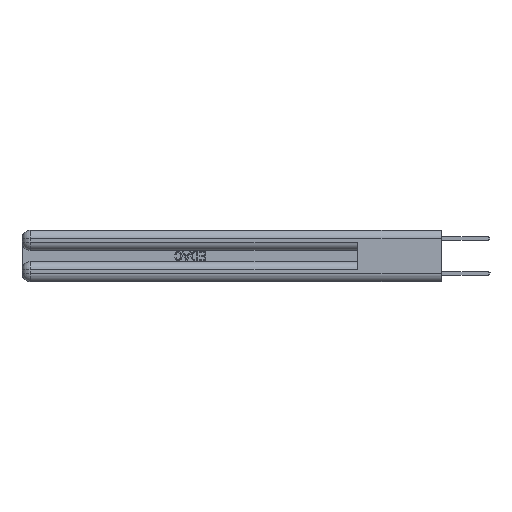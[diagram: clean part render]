
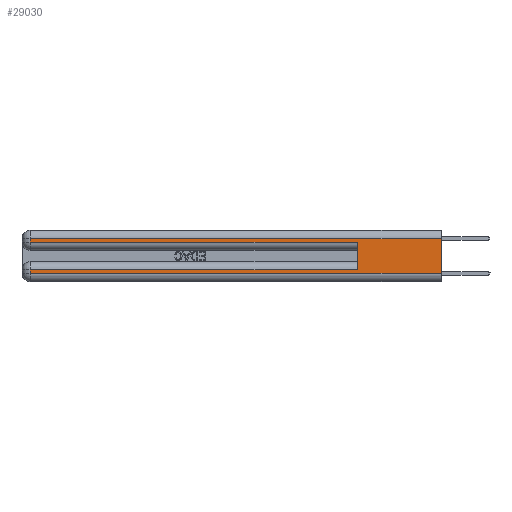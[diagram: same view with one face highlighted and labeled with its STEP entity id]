
A CAD part, left-side view. The second image highlights one B-rep face of the part: STEP entity #29030.
In plain terms, the highlighted planar face has unit normal (-1, 0, 0).
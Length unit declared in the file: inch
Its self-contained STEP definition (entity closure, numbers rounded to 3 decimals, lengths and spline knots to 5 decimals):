
#73 = EDGE_CURVE ( 'NONE', #23236, #11165, #15720, .T. ) ;
#174 = LINE ( 'NONE', #9758, #1779 ) ;
#1779 = VECTOR ( 'NONE', #19811, 39.37008 ) ;
#2543 = VERTEX_POINT ( 'NONE', #21109 ) ;
#2644 = CARTESIAN_POINT ( 'NONE',  ( 0., 2.94, 0.31 ) ) ;
#2807 = ORIENTED_EDGE ( 'NONE', *, *, #21782, .T. ) ;
#2989 = LINE ( 'NONE', #7926, #9558 ) ;
#2991 = DIRECTION ( 'NONE',  ( 0., -1., 0. ) ) ;
#3106 = VECTOR ( 'NONE', #4340, 39.37008 ) ;
#3146 = CARTESIAN_POINT ( 'NONE',  ( 0., 0., 0.37 ) ) ;
#3675 = EDGE_CURVE ( 'NONE', #23907, #11270, #6898, .T. ) ;
#4340 = DIRECTION ( 'NONE',  ( 0., 0., 1. ) ) ;
#4606 = LINE ( 'NONE', #21696, #10501 ) ;
#4812 = CARTESIAN_POINT ( 'NONE',  ( 0., 0., 0.06 ) ) ;
#5123 = AXIS2_PLACEMENT_3D ( 'NONE', #3146, #22625, #29956 ) ;
#6491 = ORIENTED_EDGE ( 'NONE', *, *, #29100, .T. ) ;
#6836 = VECTOR ( 'NONE', #2991, 39.37008 ) ;
#6898 = LINE ( 'NONE', #23993, #3106 ) ;
#7926 = CARTESIAN_POINT ( 'NONE',  ( 0., 0., 0.085 ) ) ;
#8529 = DIRECTION ( 'NONE',  ( 0., 0., -1. ) ) ;
#9203 = DIRECTION ( 'NONE',  ( 0., -1., 0. ) ) ;
#9499 = EDGE_CURVE ( 'NONE', #2543, #26102, #20677, .T. ) ;
#9523 = ORIENTED_EDGE ( 'NONE', *, *, #12808, .T. ) ;
#9558 = VECTOR ( 'NONE', #24854, 39.37008 ) ;
#9758 = CARTESIAN_POINT ( 'NONE',  ( 0., 0., 0.31 ) ) ;
#10501 = VECTOR ( 'NONE', #26626, 39.37008 ) ;
#10565 = ORIENTED_EDGE ( 'NONE', *, *, #9499, .F. ) ;
#10576 = VERTEX_POINT ( 'NONE', #14736 ) ;
#10870 = ORIENTED_EDGE ( 'NONE', *, *, #73, .T. ) ;
#11165 = VERTEX_POINT ( 'NONE', #15153 ) ;
#11270 = VERTEX_POINT ( 'NONE', #12761 ) ;
#11404 = CARTESIAN_POINT ( 'NONE',  ( 0., 0., 0.37 ) ) ;
#12761 = CARTESIAN_POINT ( 'NONE',  ( 0., 0.6, 0.285 ) ) ;
#12808 = EDGE_CURVE ( 'NONE', #23907, #23236, #2989, .T. ) ;
#13144 = VERTEX_POINT ( 'NONE', #2644 ) ;
#14317 = LINE ( 'NONE', #25949, #26524 ) ;
#14602 = CARTESIAN_POINT ( 'NONE',  ( 0., 2.94, 0.085 ) ) ;
#14736 = CARTESIAN_POINT ( 'NONE',  ( 0., 2.94, 0.285 ) ) ;
#15153 = CARTESIAN_POINT ( 'NONE',  ( 0., 2.94, 0.06 ) ) ;
#15720 = LINE ( 'NONE', #29928, #16192 ) ;
#16192 = VECTOR ( 'NONE', #8529, 39.37008 ) ;
#18207 = EDGE_CURVE ( 'NONE', #10576, #11270, #27092, .T. ) ;
#18534 = ORIENTED_EDGE ( 'NONE', *, *, #3675, .F. ) ;
#19811 = DIRECTION ( 'NONE',  ( 0., 1., 0. ) ) ;
#19926 = CARTESIAN_POINT ( 'NONE',  ( 0., 0., 0.285 ) ) ;
#20124 = EDGE_CURVE ( 'NONE', #2543, #13144, #174, .T. ) ;
#20657 = EDGE_LOOP ( 'NONE', ( #10565, #22474, #2807, #24044, #18534, #9523, #10870, #6491 ) ) ;
#20677 = LINE ( 'NONE', #11404, #28775 ) ;
#21109 = CARTESIAN_POINT ( 'NONE',  ( 0., 0., 0.31 ) ) ;
#21150 = DIRECTION ( 'NONE',  ( 0., 0., -1. ) ) ;
#21696 = CARTESIAN_POINT ( 'NONE',  ( 0., 2.94, 0.37 ) ) ;
#21782 = EDGE_CURVE ( 'NONE', #13144, #10576, #4606, .T. ) ;
#22474 = ORIENTED_EDGE ( 'NONE', *, *, #20124, .T. ) ;
#22625 = DIRECTION ( 'NONE',  ( 1., 0., 0. ) ) ;
#23236 = VERTEX_POINT ( 'NONE', #14602 ) ;
#23907 = VERTEX_POINT ( 'NONE', #30308 ) ;
#23993 = CARTESIAN_POINT ( 'NONE',  ( 0., 0.6, 0.145 ) ) ;
#24044 = ORIENTED_EDGE ( 'NONE', *, *, #18207, .T. ) ;
#24854 = DIRECTION ( 'NONE',  ( 0., 1., 0. ) ) ;
#25012 = FACE_OUTER_BOUND ( 'NONE', #20657, .T. ) ;
#25949 = CARTESIAN_POINT ( 'NONE',  ( 0., 0., 0.06 ) ) ;
#26102 = VERTEX_POINT ( 'NONE', #4812 ) ;
#26524 = VECTOR ( 'NONE', #9203, 39.37008 ) ;
#26626 = DIRECTION ( 'NONE',  ( 0., 0., -1. ) ) ;
#27092 = LINE ( 'NONE', #19926, #6836 ) ;
#27558 = PLANE ( 'NONE',  #5123 ) ;
#28775 = VECTOR ( 'NONE', #21150, 39.37008 ) ;
#29030 = ADVANCED_FACE ( 'NONE', ( #25012 ), #27558, .F. ) ;
#29100 = EDGE_CURVE ( 'NONE', #11165, #26102, #14317, .T. ) ;
#29928 = CARTESIAN_POINT ( 'NONE',  ( 0., 2.94, 0.37 ) ) ;
#29956 = DIRECTION ( 'NONE',  ( 0., 0., -1. ) ) ;
#30308 = CARTESIAN_POINT ( 'NONE',  ( 0., 0.6, 0.085 ) ) ;
